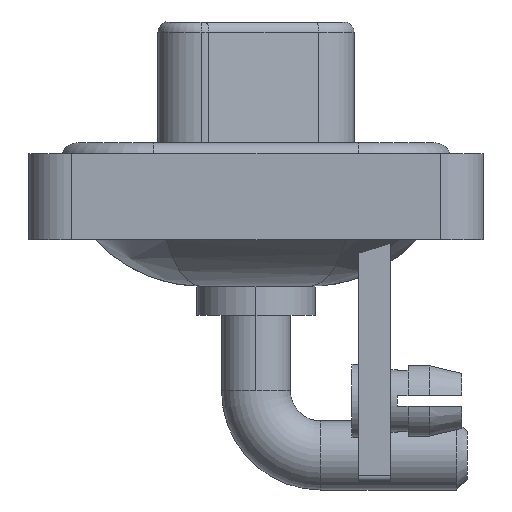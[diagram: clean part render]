
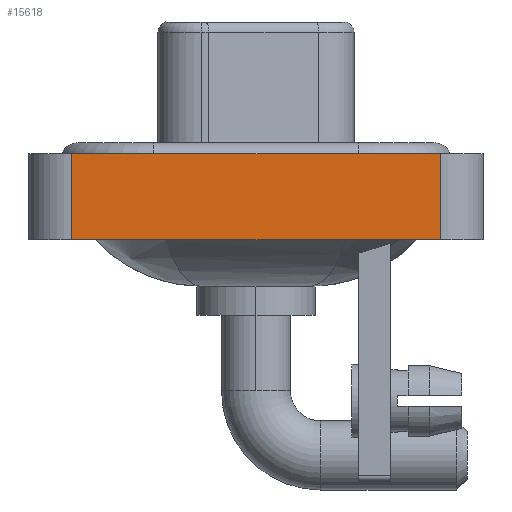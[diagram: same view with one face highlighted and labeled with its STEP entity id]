
A CAD part, left-side view. The second image highlights one B-rep face of the part: STEP entity #15618.
In plain terms, the highlighted planar face has unit normal (-1, 0, 0).
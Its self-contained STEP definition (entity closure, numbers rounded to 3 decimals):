
#305 = FACE_OUTER_BOUND ( 'NONE', #438, .T. ) ;
#373 = AXIS2_PLACEMENT_3D ( 'NONE', #12133, #6120, #12046 ) ;
#438 = EDGE_LOOP ( 'NONE', ( #18283, #18522, #8539, #3135 ) ) ;
#874 = CARTESIAN_POINT ( 'NONE',  ( -7.3, -8.55, -3.6 ) ) ;
#1151 = DIRECTION ( 'NONE',  ( 0., -1., 0. ) ) ;
#2685 = EDGE_CURVE ( 'NONE', #5727, #12516, #11469, .T. ) ;
#3135 = ORIENTED_EDGE ( 'NONE', *, *, #14502, .T. ) ;
#4257 = CARTESIAN_POINT ( 'NONE',  ( -7.3, 8.55, -3.6 ) ) ;
#5199 = VECTOR ( 'NONE', #11478, 1000. ) ;
#5727 = VERTEX_POINT ( 'NONE', #7900 ) ;
#6120 = DIRECTION ( 'NONE',  ( -1., 0., 0. ) ) ;
#6178 = VECTOR ( 'NONE', #13908, 1000. ) ;
#6214 = PLANE ( 'NONE',  #373 ) ;
#7071 = VERTEX_POINT ( 'NONE', #4257 ) ;
#7368 = DIRECTION ( 'NONE',  ( 0., -1., 0. ) ) ;
#7900 = CARTESIAN_POINT ( 'NONE',  ( -7.3, 8.55, 0.4 ) ) ;
#8344 = CARTESIAN_POINT ( 'NONE',  ( -7.3, 8.55, -3.6 ) ) ;
#8539 = ORIENTED_EDGE ( 'NONE', *, *, #17954, .F. ) ;
#9288 = VECTOR ( 'NONE', #1151, 1000. ) ;
#9790 = LINE ( 'NONE', #8344, #6178 ) ;
#9835 = CARTESIAN_POINT ( 'NONE',  ( -7.3, -8.55, 0.4 ) ) ;
#10056 = LINE ( 'NONE', #10160, #17688 ) ;
#10160 = CARTESIAN_POINT ( 'NONE',  ( -7.3, -8.55, -3.6 ) ) ;
#11469 = LINE ( 'NONE', #9835, #9288 ) ;
#11478 = DIRECTION ( 'NONE',  ( 0., 0., 1. ) ) ;
#12046 = DIRECTION ( 'NONE',  ( 0., 0., 1. ) ) ;
#12133 = CARTESIAN_POINT ( 'NONE',  ( -7.3, -8.55, -3.6 ) ) ;
#12245 = CARTESIAN_POINT ( 'NONE',  ( -7.3, -8.55, -3.6 ) ) ;
#12414 = VERTEX_POINT ( 'NONE', #12245 ) ;
#12516 = VERTEX_POINT ( 'NONE', #18157 ) ;
#13908 = DIRECTION ( 'NONE',  ( 0., 0., 1. ) ) ;
#14502 = EDGE_CURVE ( 'NONE', #7071, #12414, #10056, .T. ) ;
#15582 = LINE ( 'NONE', #874, #5199 ) ;
#15618 = ADVANCED_FACE ( 'NONE', ( #305 ), #6214, .T. ) ;
#16668 = EDGE_CURVE ( 'NONE', #12414, #12516, #15582, .T. ) ;
#17688 = VECTOR ( 'NONE', #7368, 1000. ) ;
#17954 = EDGE_CURVE ( 'NONE', #7071, #5727, #9790, .T. ) ;
#18157 = CARTESIAN_POINT ( 'NONE',  ( -7.3, -8.55, 0.4 ) ) ;
#18283 = ORIENTED_EDGE ( 'NONE', *, *, #16668, .T. ) ;
#18522 = ORIENTED_EDGE ( 'NONE', *, *, #2685, .F. ) ;
